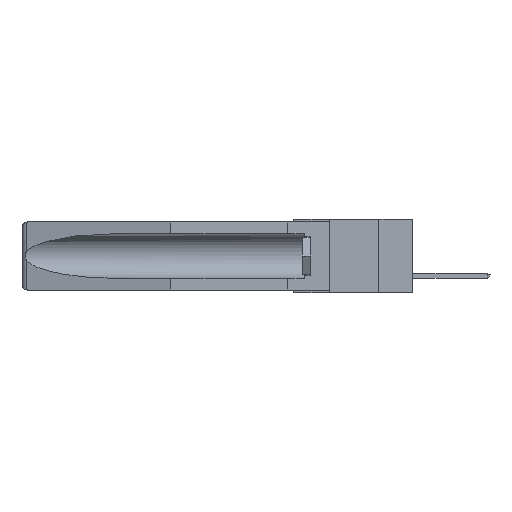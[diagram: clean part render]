
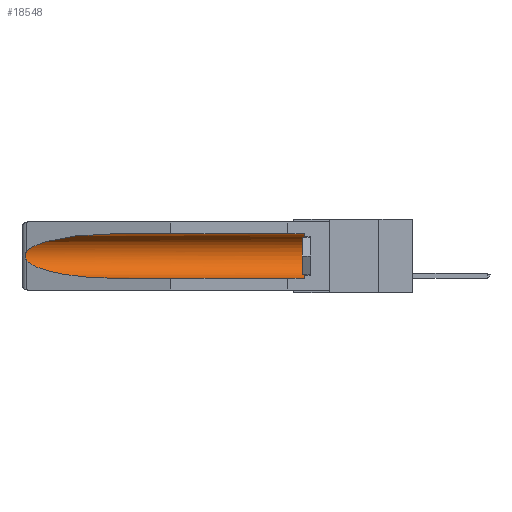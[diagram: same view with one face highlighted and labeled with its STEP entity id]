
A CAD part, left-side view. The second image highlights one B-rep face of the part: STEP entity #18548.
In plain terms, the highlighted cylindrical face has radius 2.857 mm (diameter 5.715 mm), a partial arc.
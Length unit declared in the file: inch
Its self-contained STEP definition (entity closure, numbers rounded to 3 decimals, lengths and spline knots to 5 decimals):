
#9 = B_SPLINE_CURVE_WITH_KNOTS ( 'NONE', 3,
 ( #9182, #12241, #3218, #17525, #12966, #10180, #1128, #11558, #13319, #5654 ),
 .UNSPECIFIED., .F., .F.,
 ( 4, 2, 2, 2, 4 ),
 ( 0., 0.00029, 0.00058, 0.00087, 0.00117 ),
 .UNSPECIFIED. ) ;
#358 = EDGE_CURVE ( 'NONE', #7825, #3958, #612, .T. ) ;
#612 = CIRCLE ( 'NONE', #15261, 0.1125 ) ;
#654 = DIRECTION ( 'NONE',  ( 0., 1., 0. ) ) ;
#698 = EDGE_LOOP ( 'NONE', ( #3006, #11053, #13500, #5070, #10589, #2969 ) ) ;
#1128 = CARTESIAN_POINT ( 'NONE',  ( 0.2673, 1.53269, -0.17917 ) ) ;
#1877 =( BOUNDED_CURVE ( )  B_SPLINE_CURVE ( 3, ( #12390, #18742, #18495, #2065 ),
 .UNSPECIFIED., .F., .F. ) 
 B_SPLINE_CURVE_WITH_KNOTS ( ( 4, 4 ),
 ( 0.1948, 1.5708 ),
 .UNSPECIFIED. ) 
 CURVE ( )  GEOMETRIC_REPRESENTATION_ITEM ( )  RATIONAL_B_SPLINE_CURVE ( ( 1., 0.848, 0.848, 1. ) ) 
 REPRESENTATION_ITEM ( '' )  );
#1895 = CARTESIAN_POINT ( 'NONE',  ( 0.155, 0.126, -0.1715 ) ) ;
#2065 = CARTESIAN_POINT ( 'NONE',  ( 0.155, 1.07973, -0.284 ) ) ;
#2072 = DIRECTION ( 'NONE',  ( 0., 0., 1. ) ) ;
#2225 = EDGE_CURVE ( 'NONE', #3958, #12689, #4585, .T. ) ;
#2896 = CARTESIAN_POINT ( 'NONE',  ( 0.155, -0.30754, -0.284 ) ) ;
#2969 = ORIENTED_EDGE ( 'NONE', *, *, #2225, .T. ) ;
#3006 = ORIENTED_EDGE ( 'NONE', *, *, #14642, .T. ) ;
#3218 = CARTESIAN_POINT ( 'NONE',  ( 0.26654, 1.53092, -0.15636 ) ) ;
#3450 = DIRECTION ( 'NONE',  ( 0., -1., 0. ) ) ;
#3826 = CARTESIAN_POINT ( 'NONE',  ( 0.155, -0.30754, -0.059 ) ) ;
#3880 = CARTESIAN_POINT ( 'NONE',  ( 0.21114, 1.30732, -0.059 ) ) ;
#3958 = VERTEX_POINT ( 'NONE', #8069 ) ;
#4501 = VERTEX_POINT ( 'NONE', #19635 ) ;
#4585 = LINE ( 'NONE', #3826, #16248 ) ;
#5062 = VECTOR ( 'NONE', #14817, 39.37008 ) ;
#5070 = ORIENTED_EDGE ( 'NONE', *, *, #14723, .F. ) ;
#5654 = CARTESIAN_POINT ( 'NONE',  ( 0.26537, 1.52718, -0.19328 ) ) ;
#6560 = VERTEX_POINT ( 'NONE', #14337 ) ;
#6928 = CARTESIAN_POINT ( 'NONE',  ( 0.25451, 1.48313, -0.09465 ) ) ;
#7577 = EDGE_CURVE ( 'NONE', #4501, #6560, #9, .T. ) ;
#7825 = VERTEX_POINT ( 'NONE', #19057 ) ;
#8069 = CARTESIAN_POINT ( 'NONE',  ( 0.155, 0.126, -0.059 ) ) ;
#8119 = DIRECTION ( 'NONE',  ( 0., 0., 1. ) ) ;
#9039 = VERTEX_POINT ( 'NONE', #17620 ) ;
#9182 = CARTESIAN_POINT ( 'NONE',  ( 0.26537, 1.52718, -0.14972 ) ) ;
#10059 = LINE ( 'NONE', #2896, #5062 ) ;
#10180 = CARTESIAN_POINT ( 'NONE',  ( 0.2675, 1.53308, -0.17534 ) ) ;
#10589 = ORIENTED_EDGE ( 'NONE', *, *, #358, .T. ) ;
#11053 = ORIENTED_EDGE ( 'NONE', *, *, #7577, .T. ) ;
#11558 = CARTESIAN_POINT ( 'NONE',  ( 0.26655, 1.53094, -0.18657 ) ) ;
#11660 = EDGE_CURVE ( 'NONE', #6560, #9039, #1877, .T. ) ;
#11899 = CARTESIAN_POINT ( 'NONE',  ( 0.155, 1.07973, -0.059 ) ) ;
#12241 = CARTESIAN_POINT ( 'NONE',  ( 0.26597, 1.52961, -0.15275 ) ) ;
#12390 = CARTESIAN_POINT ( 'NONE',  ( 0.26537, 1.52718, -0.19328 ) ) ;
#12689 = VERTEX_POINT ( 'NONE', #11899 ) ;
#12966 = CARTESIAN_POINT ( 'NONE',  ( 0.2675, 1.53308, -0.16763 ) ) ;
#13319 = CARTESIAN_POINT ( 'NONE',  ( 0.26597, 1.5296, -0.19026 ) ) ;
#13500 = ORIENTED_EDGE ( 'NONE', *, *, #11660, .T. ) ;
#13584 = FACE_OUTER_BOUND ( 'NONE', #698, .T. ) ;
#14337 = CARTESIAN_POINT ( 'NONE',  ( 0.26537, 1.52718, -0.19328 ) ) ;
#14642 = EDGE_CURVE ( 'NONE', #12689, #4501, #18901, .T. ) ;
#14689 = CARTESIAN_POINT ( 'NONE',  ( 0.26537, 1.52718, -0.14972 ) ) ;
#14723 = EDGE_CURVE ( 'NONE', #7825, #9039, #10059, .T. ) ;
#14798 = CYLINDRICAL_SURFACE ( 'NONE', #15085, 0.1125 ) ;
#14817 = DIRECTION ( 'NONE',  ( 0., 1., 0. ) ) ;
#15085 = AXIS2_PLACEMENT_3D ( 'NONE', #17216, #654, #2072 ) ;
#15261 = AXIS2_PLACEMENT_3D ( 'NONE', #1895, #3450, #8119 ) ;
#16248 = VECTOR ( 'NONE', #19150, 39.37008 ) ;
#17154 = CARTESIAN_POINT ( 'NONE',  ( 0.155, 1.07973, -0.059 ) ) ;
#17216 = CARTESIAN_POINT ( 'NONE',  ( 0.155, -0.30754, -0.1715 ) ) ;
#17525 = CARTESIAN_POINT ( 'NONE',  ( 0.2673, 1.5327, -0.16383 ) ) ;
#17620 = CARTESIAN_POINT ( 'NONE',  ( 0.155, 1.07973, -0.284 ) ) ;
#18495 = CARTESIAN_POINT ( 'NONE',  ( 0.21114, 1.30732, -0.284 ) ) ;
#18548 = ADVANCED_FACE ( 'NONE', ( #13584 ), #14798, .F. ) ;
#18742 = CARTESIAN_POINT ( 'NONE',  ( 0.25451, 1.48313, -0.24835 ) ) ;
#18901 =( BOUNDED_CURVE ( )  B_SPLINE_CURVE ( 3, ( #17154, #3880, #6928, #14689 ),
 .UNSPECIFIED., .F., .F. ) 
 B_SPLINE_CURVE_WITH_KNOTS ( ( 4, 4 ),
 ( 4.71239, 6.08839 ),
 .UNSPECIFIED. ) 
 CURVE ( )  GEOMETRIC_REPRESENTATION_ITEM ( )  RATIONAL_B_SPLINE_CURVE ( ( 1., 0.848, 0.848, 1. ) ) 
 REPRESENTATION_ITEM ( '' )  );
#19057 = CARTESIAN_POINT ( 'NONE',  ( 0.155, 0.126, -0.284 ) ) ;
#19150 = DIRECTION ( 'NONE',  ( 0., 1., 0. ) ) ;
#19635 = CARTESIAN_POINT ( 'NONE',  ( 0.26537, 1.52718, -0.14972 ) ) ;
